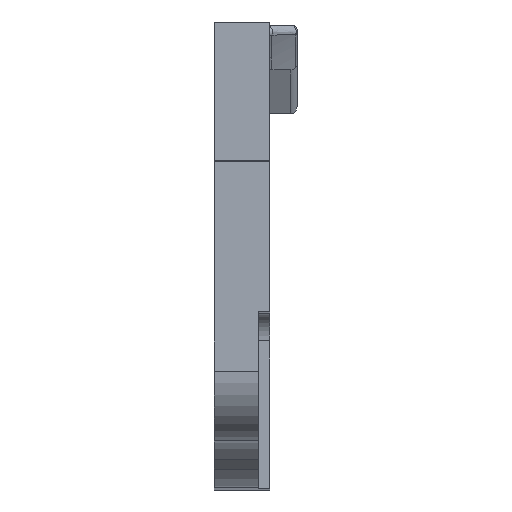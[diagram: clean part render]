
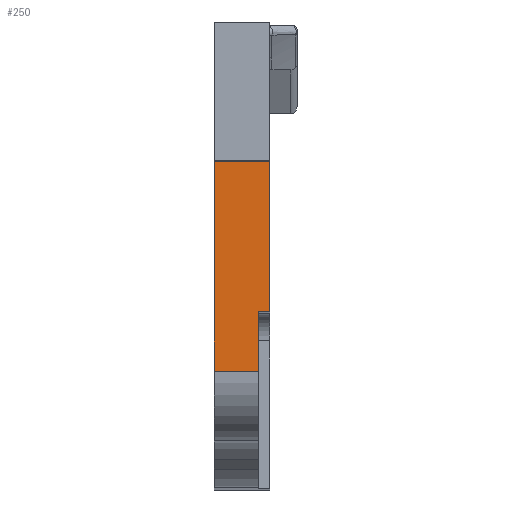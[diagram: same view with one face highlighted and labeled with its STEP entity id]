
A CAD part, top view. The second image highlights one B-rep face of the part: STEP entity #250.
In plain terms, the highlighted planar face has unit normal (0, 0, 1).
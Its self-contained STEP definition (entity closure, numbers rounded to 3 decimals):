
#23 = EDGE_CURVE ( 'NONE', #105, #2884, #1235, .T. ) ;
#27 = CARTESIAN_POINT ( 'NONE',  ( 28.082, 8.346, 3.82 ) ) ;
#105 = VERTEX_POINT ( 'NONE', #1677 ) ;
#195 = DIRECTION ( 'NONE',  ( 0., 1., 0. ) ) ;
#231 = VECTOR ( 'NONE', #2359, 1000. ) ;
#250 = ADVANCED_FACE ( 'NONE', ( #4123 ), #3877, .T. ) ;
#278 = AXIS2_PLACEMENT_3D ( 'NONE', #1210, #3902, #480 ) ;
#291 = LINE ( 'NONE', #3631, #1201 ) ;
#343 = ORIENTED_EDGE ( 'NONE', *, *, #1958, .F. ) ;
#350 = VECTOR ( 'NONE', #418, 1000. ) ;
#418 = DIRECTION ( 'NONE',  ( 1., 0., 0. ) ) ;
#480 = DIRECTION ( 'NONE',  ( 1., 0., 0. ) ) ;
#585 = ORIENTED_EDGE ( 'NONE', *, *, #3737, .T. ) ;
#664 = CARTESIAN_POINT ( 'NONE',  ( 4., 12.63, 3.82 ) ) ;
#951 = CARTESIAN_POINT ( 'NONE',  ( 0., 3.346, 3.82 ) ) ;
#963 = VERTEX_POINT ( 'NONE', #2487 ) ;
#1066 = CARTESIAN_POINT ( 'NONE',  ( 3.175, 12.63, 3.82 ) ) ;
#1088 = CARTESIAN_POINT ( 'NONE',  ( 3.175, 12.63, 3.82 ) ) ;
#1139 = VERTEX_POINT ( 'NONE', #664 ) ;
#1201 = VECTOR ( 'NONE', #1590, 1000. ) ;
#1210 = CARTESIAN_POINT ( 'NONE',  ( 28.082, 3.346, 3.82 ) ) ;
#1235 = LINE ( 'NONE', #2249, #3224 ) ;
#1281 = EDGE_CURVE ( 'NONE', #3366, #1139, #3797, .T. ) ;
#1359 = ORIENTED_EDGE ( 'NONE', *, *, #23, .T. ) ;
#1432 = DIRECTION ( 'NONE',  ( 0., 1., 0. ) ) ;
#1486 = ORIENTED_EDGE ( 'NONE', *, *, #1281, .T. ) ;
#1590 = DIRECTION ( 'NONE',  ( 0., -1., 0. ) ) ;
#1614 = EDGE_LOOP ( 'NONE', ( #1486, #2406, #1359, #343, #585, #3788 ) ) ;
#1618 = DIRECTION ( 'NONE',  ( -1., 0., 0. ) ) ;
#1677 = CARTESIAN_POINT ( 'NONE',  ( 4., 23.446, 3.82 ) ) ;
#1720 = LINE ( 'NONE', #2424, #2129 ) ;
#1958 = EDGE_CURVE ( 'NONE', #2098, #2884, #3973, .T. ) ;
#1998 = EDGE_CURVE ( 'NONE', #3366, #963, #291, .T. ) ;
#2049 = VECTOR ( 'NONE', #195, 1000. ) ;
#2098 = VERTEX_POINT ( 'NONE', #3490 ) ;
#2129 = VECTOR ( 'NONE', #1432, 1000. ) ;
#2249 = CARTESIAN_POINT ( 'NONE',  ( 10., 23.446, 3.82 ) ) ;
#2359 = DIRECTION ( 'NONE',  ( 1., 0., 0. ) ) ;
#2406 = ORIENTED_EDGE ( 'NONE', *, *, #4161, .T. ) ;
#2424 = CARTESIAN_POINT ( 'NONE',  ( 4., 3.346, 3.82 ) ) ;
#2487 = CARTESIAN_POINT ( 'NONE',  ( 3.175, 8.346, 3.82 ) ) ;
#2870 = CARTESIAN_POINT ( 'NONE',  ( 0., 23.446, 3.82 ) ) ;
#2884 = VERTEX_POINT ( 'NONE', #2870 ) ;
#3067 = LINE ( 'NONE', #27, #231 ) ;
#3224 = VECTOR ( 'NONE', #1618, 1000. ) ;
#3366 = VERTEX_POINT ( 'NONE', #1066 ) ;
#3490 = CARTESIAN_POINT ( 'NONE',  ( 0., 8.346, 3.82 ) ) ;
#3631 = CARTESIAN_POINT ( 'NONE',  ( 3.175, 8.346, 3.82 ) ) ;
#3737 = EDGE_CURVE ( 'NONE', #2098, #963, #3067, .T. ) ;
#3788 = ORIENTED_EDGE ( 'NONE', *, *, #1998, .F. ) ;
#3797 = LINE ( 'NONE', #1088, #350 ) ;
#3877 = PLANE ( 'NONE',  #278 ) ;
#3902 = DIRECTION ( 'NONE',  ( 0., 0., 1. ) ) ;
#3973 = LINE ( 'NONE', #951, #2049 ) ;
#4123 = FACE_OUTER_BOUND ( 'NONE', #1614, .T. ) ;
#4161 = EDGE_CURVE ( 'NONE', #1139, #105, #1720, .T. ) ;
